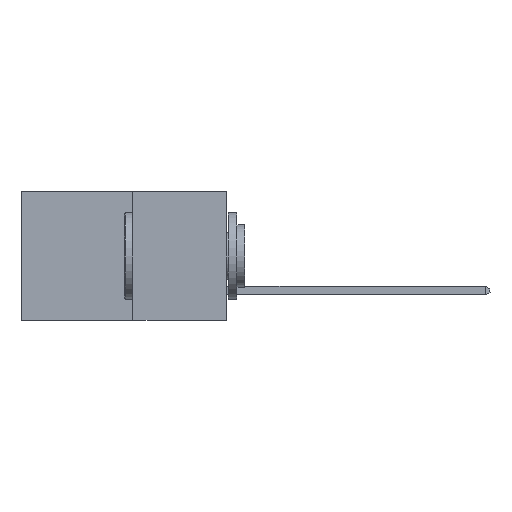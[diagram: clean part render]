
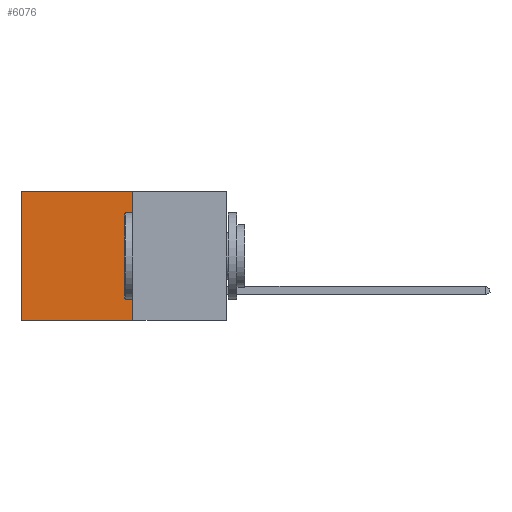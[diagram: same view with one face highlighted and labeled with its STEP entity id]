
A CAD part, left-side view. The second image highlights one B-rep face of the part: STEP entity #6076.
In plain terms, the highlighted planar face has unit normal (-1, 0, 0).
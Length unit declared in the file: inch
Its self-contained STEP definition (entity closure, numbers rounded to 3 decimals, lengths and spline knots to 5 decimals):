
#1265 = CARTESIAN_POINT ( 'NONE',  ( 0.277, 0.59, 0. ) ) ;
#1481 = DIRECTION ( 'NONE',  ( 0., 0., -1. ) ) ;
#1590 = DIRECTION ( 'NONE',  ( 0., 1., 0. ) ) ;
#2334 = CARTESIAN_POINT ( 'NONE',  ( 0.277, 0.59, -0.37 ) ) ;
#2396 = VERTEX_POINT ( 'NONE', #7771 ) ;
#4046 = ORIENTED_EDGE ( 'NONE', *, *, #5907, .F. ) ;
#4308 = VERTEX_POINT ( 'NONE', #2334 ) ;
#5201 = AXIS2_PLACEMENT_3D ( 'NONE', #8707, #8624, #8591 ) ;
#5292 = CARTESIAN_POINT ( 'NONE',  ( 0.277, 0.59, -0.37 ) ) ;
#5907 = EDGE_CURVE ( 'NONE', #2396, #4308, #10960, .T. ) ;
#6076 = ADVANCED_FACE ( 'NONE', ( #11821 ), #8946, .F. ) ;
#7771 = CARTESIAN_POINT ( 'NONE',  ( 0.277, 0.27, -0.37 ) ) ;
#8591 = DIRECTION ( 'NONE',  ( 0., 0., -1. ) ) ;
#8624 = DIRECTION ( 'NONE',  ( 1., 0., 0. ) ) ;
#8707 = CARTESIAN_POINT ( 'NONE',  ( 0.277, 0.27, -0.37 ) ) ;
#8946 = PLANE ( 'NONE',  #5201 ) ;
#9332 = LINE ( 'NONE', #5292, #23145 ) ;
#9571 = CARTESIAN_POINT ( 'NONE',  ( 0.277, 0.27, -0.37 ) ) ;
#10670 = EDGE_CURVE ( 'NONE', #16439, #20553, #11092, .T. ) ;
#10960 = LINE ( 'NONE', #11566, #14778 ) ;
#11031 = DIRECTION ( 'NONE',  ( 0., 1., 0. ) ) ;
#11092 = LINE ( 'NONE', #22451, #21131 ) ;
#11366 = DIRECTION ( 'NONE',  ( 0., 0., -1. ) ) ;
#11566 = CARTESIAN_POINT ( 'NONE',  ( 0.277, 0.27, -0.37 ) ) ;
#11821 = FACE_OUTER_BOUND ( 'NONE', #16562, .T. ) ;
#12045 = VECTOR ( 'NONE', #11366, 39.37008 ) ;
#13150 = ORIENTED_EDGE ( 'NONE', *, *, #18229, .F. ) ;
#14479 = EDGE_CURVE ( 'NONE', #20553, #4308, #9332, .T. ) ;
#14778 = VECTOR ( 'NONE', #11031, 39.37008 ) ;
#16439 = VERTEX_POINT ( 'NONE', #20845 ) ;
#16562 = EDGE_LOOP ( 'NONE', ( #19695, #4046, #13150, #21432 ) ) ;
#18229 = EDGE_CURVE ( 'NONE', #16439, #2396, #22084, .T. ) ;
#19695 = ORIENTED_EDGE ( 'NONE', *, *, #14479, .T. ) ;
#20553 = VERTEX_POINT ( 'NONE', #1265 ) ;
#20845 = CARTESIAN_POINT ( 'NONE',  ( 0.277, 0.27, 0. ) ) ;
#21131 = VECTOR ( 'NONE', #1590, 39.37008 ) ;
#21432 = ORIENTED_EDGE ( 'NONE', *, *, #10670, .T. ) ;
#22084 = LINE ( 'NONE', #9571, #12045 ) ;
#22451 = CARTESIAN_POINT ( 'NONE',  ( 0.277, 0.27, 0. ) ) ;
#23145 = VECTOR ( 'NONE', #1481, 39.37008 ) ;
